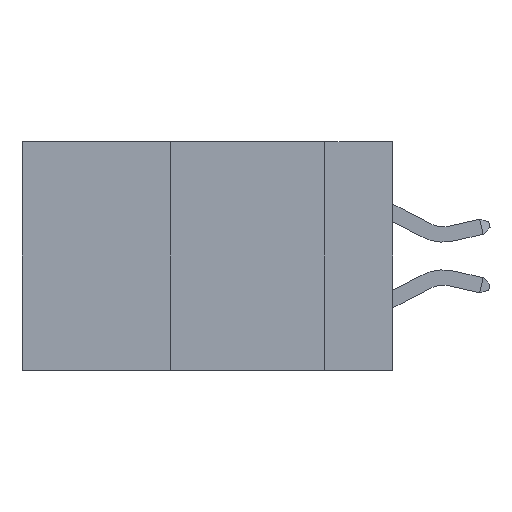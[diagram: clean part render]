
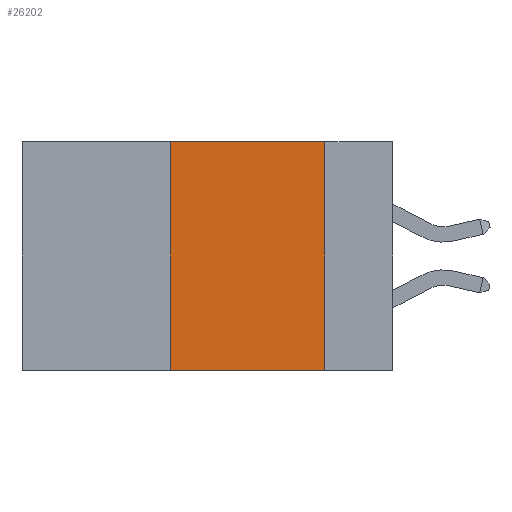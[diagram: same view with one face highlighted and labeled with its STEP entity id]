
A CAD part, left-side view. The second image highlights one B-rep face of the part: STEP entity #26202.
In plain terms, the highlighted planar face has unit normal (-1, 0, 0).
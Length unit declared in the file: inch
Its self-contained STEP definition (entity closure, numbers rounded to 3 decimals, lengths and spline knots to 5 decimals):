
#236 = EDGE_CURVE ( 'NONE', #5931, #10950, #26385, .T. ) ;
#1955 = CARTESIAN_POINT ( 'NONE',  ( 0., 0.6, -0.37 ) ) ;
#2803 = LINE ( 'NONE', #27615, #13931 ) ;
#3953 = ORIENTED_EDGE ( 'NONE', *, *, #8972, .F. ) ;
#4565 = CARTESIAN_POINT ( 'NONE',  ( 0., 0.11, -0.37 ) ) ;
#5931 = VERTEX_POINT ( 'NONE', #12683 ) ;
#6492 = VERTEX_POINT ( 'NONE', #24801 ) ;
#7688 = CARTESIAN_POINT ( 'NONE',  ( 0., 0.6, 0. ) ) ;
#7812 = DIRECTION ( 'NONE',  ( 0., -1., 0. ) ) ;
#8972 = EDGE_CURVE ( 'NONE', #6492, #18112, #22202, .T. ) ;
#9306 = EDGE_LOOP ( 'NONE', ( #25874, #3953, #14295, #14744 ) ) ;
#10950 = VERTEX_POINT ( 'NONE', #4565 ) ;
#11075 = EDGE_CURVE ( 'NONE', #18112, #10950, #25831, .T. ) ;
#12594 = EDGE_CURVE ( 'NONE', #5931, #6492, #2803, .T. ) ;
#12683 = CARTESIAN_POINT ( 'NONE',  ( 0., 0.36, -0.37 ) ) ;
#13931 = VECTOR ( 'NONE', #23315, 39.37008 ) ;
#14167 = DIRECTION ( 'NONE',  ( 1., 0., 0. ) ) ;
#14295 = ORIENTED_EDGE ( 'NONE', *, *, #12594, .F. ) ;
#14712 = VECTOR ( 'NONE', #24912, 39.37008 ) ;
#14744 = ORIENTED_EDGE ( 'NONE', *, *, #236, .T. ) ;
#15190 = DIRECTION ( 'NONE',  ( 0., -1., 0. ) ) ;
#16302 = VECTOR ( 'NONE', #7812, 39.37008 ) ;
#16612 = FACE_OUTER_BOUND ( 'NONE', #9306, .T. ) ;
#18112 = VERTEX_POINT ( 'NONE', #25658 ) ;
#18501 = CARTESIAN_POINT ( 'NONE',  ( 0., 0.11, 0. ) ) ;
#18657 = CARTESIAN_POINT ( 'NONE',  ( 0., 0.6, 0. ) ) ;
#20467 = VECTOR ( 'NONE', #15190, 39.37008 ) ;
#20548 = AXIS2_PLACEMENT_3D ( 'NONE', #7688, #14167, #25140 ) ;
#22202 = LINE ( 'NONE', #18657, #16302 ) ;
#22898 = PLANE ( 'NONE',  #20548 ) ;
#23315 = DIRECTION ( 'NONE',  ( 0., 0., 1. ) ) ;
#24801 = CARTESIAN_POINT ( 'NONE',  ( 0., 0.36, 0. ) ) ;
#24912 = DIRECTION ( 'NONE',  ( 0., 0., -1. ) ) ;
#25140 = DIRECTION ( 'NONE',  ( 0., 0., -1. ) ) ;
#25658 = CARTESIAN_POINT ( 'NONE',  ( 0., 0.11, 0. ) ) ;
#25831 = LINE ( 'NONE', #18501, #14712 ) ;
#25874 = ORIENTED_EDGE ( 'NONE', *, *, #11075, .F. ) ;
#26202 = ADVANCED_FACE ( 'NONE', ( #16612 ), #22898, .F. ) ;
#26385 = LINE ( 'NONE', #1955, #20467 ) ;
#27615 = CARTESIAN_POINT ( 'NONE',  ( 0., 0.36, 0. ) ) ;
